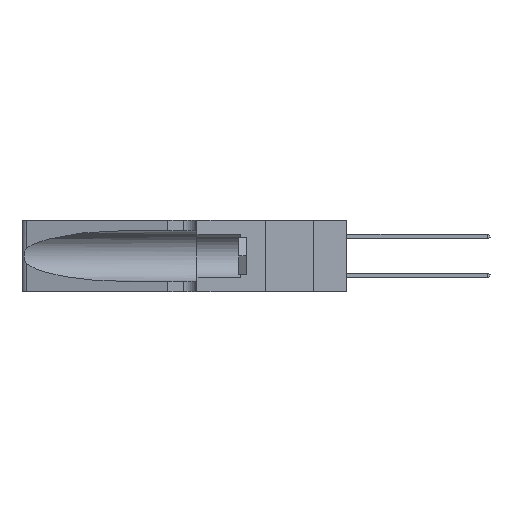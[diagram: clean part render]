
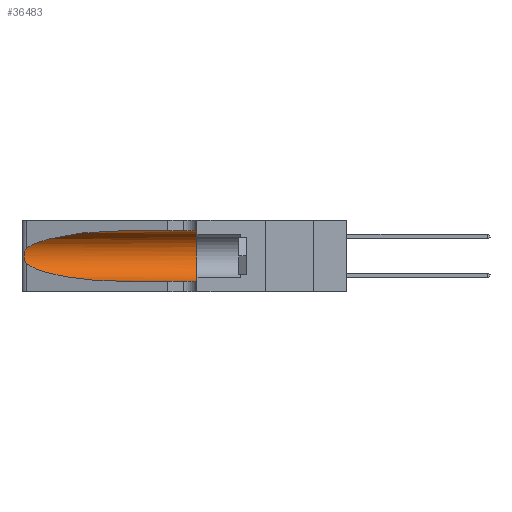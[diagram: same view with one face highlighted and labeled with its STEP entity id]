
A CAD part, left-side view. The second image highlights one B-rep face of the part: STEP entity #36483.
In plain terms, the highlighted cylindrical face has radius 3.308 mm (diameter 6.617 mm), a partial arc.
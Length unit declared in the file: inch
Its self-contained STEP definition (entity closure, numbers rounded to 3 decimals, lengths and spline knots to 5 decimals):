
#464 = CARTESIAN_POINT ( 'NONE',  ( 0.25787, 1.23484, 0.2124 ) ) ;
#1125 = EDGE_CURVE ( 'NONE', #40027, #24316, #21915, .T. ) ;
#1671 = DIRECTION ( 'NONE',  ( 0., 0., -1. ) ) ;
#1837 = CARTESIAN_POINT ( 'NONE',  ( 0.25487, 1.22718, 0.22369 ) ) ;
#2092 = ORIENTED_EDGE ( 'NONE', *, *, #38889, .T. ) ;
#2293 = CARTESIAN_POINT ( 'NONE',  ( 0.1305, 0.35, 0.31525 ) ) ;
#3446 = ORIENTED_EDGE ( 'NONE', *, *, #42935, .T. ) ;
#3939 = CARTESIAN_POINT ( 'NONE',  ( 0.26018, 1.23835, 0.19895 ) ) ;
#4341 = CARTESIAN_POINT ( 'NONE',  ( 0.18966, 0.96281, 0.05475 ) ) ;
#5694 = EDGE_CURVE ( 'NONE', #40027, #6744, #12491, .T. ) ;
#5858 = EDGE_LOOP ( 'NONE', ( #23459, #6784, #3446, #2092, #9388, #17272 ) ) ;
#5968 =( BOUNDED_CURVE ( )  B_SPLINE_CURVE ( 3, ( #17790, #37858, #4341, #27891 ),
 .UNSPECIFIED., .F., .T. ) 
 B_SPLINE_CURVE_WITH_KNOTS ( ( 4, 4 ),
 ( 3.44316, 4.71239 ),
 .UNSPECIFIED. ) 
 CURVE ( )  GEOMETRIC_REPRESENTATION_ITEM ( )  RATIONAL_B_SPLINE_CURVE ( ( 1., 0.87, 0.87, 1. ) ) 
 REPRESENTATION_ITEM ( '' )  );
#6744 = VERTEX_POINT ( 'NONE', #41160 ) ;
#6784 = ORIENTED_EDGE ( 'NONE', *, *, #17450, .T. ) ;
#7331 = VERTEX_POINT ( 'NONE', #17408 ) ;
#7383 = CARTESIAN_POINT ( 'NONE',  ( 0.26075, 1.23896, 0.178 ) ) ;
#9388 = ORIENTED_EDGE ( 'NONE', *, *, #13090, .F. ) ;
#10793 = CARTESIAN_POINT ( 'NONE',  ( 0.25856, 1.23593, 0.16098 ) ) ;
#11175 = CARTESIAN_POINT ( 'NONE',  ( 0.25487, 1.22718, 0.14631 ) ) ;
#12491 =( BOUNDED_CURVE ( )  B_SPLINE_CURVE ( 3, ( #22153, #35436, #28716, #1837 ),
 .UNSPECIFIED., .F., .F. ) 
 B_SPLINE_CURVE_WITH_KNOTS ( ( 4, 4 ),
 ( 1.5708, 2.84003 ),
 .UNSPECIFIED. ) 
 CURVE ( )  GEOMETRIC_REPRESENTATION_ITEM ( )  RATIONAL_B_SPLINE_CURVE ( ( 1., 0.87, 0.87, 1. ) ) 
 REPRESENTATION_ITEM ( '' )  );
#12757 = CARTESIAN_POINT ( 'NONE',  ( 0.1305, 0.35, 0.185 ) ) ;
#13090 = EDGE_CURVE ( 'NONE', #24316, #29160, #30477, .T. ) ;
#13878 = CARTESIAN_POINT ( 'NONE',  ( 0.1305, 1.61858, 0.31525 ) ) ;
#14041 = CYLINDRICAL_SURFACE ( 'NONE', #29720, 0.13025 ) ;
#14158 = CARTESIAN_POINT ( 'NONE',  ( 0.25639, 1.23186, 0.15144 ) ) ;
#14330 = VECTOR ( 'NONE', #26242, 39.37008 ) ;
#14621 = VERTEX_POINT ( 'NONE', #11175 ) ;
#15208 = DIRECTION ( 'NONE',  ( 0., -1., 0. ) ) ;
#15244 = CARTESIAN_POINT ( 'NONE',  ( 0.1305, 0.35, 0.05475 ) ) ;
#16123 = DIRECTION ( 'NONE',  ( 0., 0., 1. ) ) ;
#17130 = DIRECTION ( 'NONE',  ( 0., -1., 0. ) ) ;
#17272 = ORIENTED_EDGE ( 'NONE', *, *, #1125, .F. ) ;
#17408 = CARTESIAN_POINT ( 'NONE',  ( 0.1305, 0.72297, 0.05475 ) ) ;
#17410 = CARTESIAN_POINT ( 'NONE',  ( 0.25487, 1.22718, 0.22369 ) ) ;
#17450 = EDGE_CURVE ( 'NONE', #6744, #14621, #32653, .T. ) ;
#17561 = CARTESIAN_POINT ( 'NONE',  ( 0.25487, 1.22718, 0.14631 ) ) ;
#17790 = CARTESIAN_POINT ( 'NONE',  ( 0.25487, 1.22718, 0.14631 ) ) ;
#20792 = CARTESIAN_POINT ( 'NONE',  ( 0.25639, 1.23184, 0.21858 ) ) ;
#21655 = CARTESIAN_POINT ( 'NONE',  ( 0.1305, 0.72297, 0.31525 ) ) ;
#21915 = LINE ( 'NONE', #13878, #32929 ) ;
#21982 = CARTESIAN_POINT ( 'NONE',  ( 0.1305, 1.61858, 0.185 ) ) ;
#22153 = CARTESIAN_POINT ( 'NONE',  ( 0.1305, 0.72297, 0.31525 ) ) ;
#22919 = CARTESIAN_POINT ( 'NONE',  ( 0.1305, 1.61858, 0.05475 ) ) ;
#23459 = ORIENTED_EDGE ( 'NONE', *, *, #5694, .T. ) ;
#24155 = CARTESIAN_POINT ( 'NONE',  ( 0.25854, 1.2359, 0.20912 ) ) ;
#24316 = VERTEX_POINT ( 'NONE', #2293 ) ;
#26242 = DIRECTION ( 'NONE',  ( 0., -1., 0. ) ) ;
#27503 = CARTESIAN_POINT ( 'NONE',  ( 0.26075, 1.23896, 0.19203 ) ) ;
#27891 = CARTESIAN_POINT ( 'NONE',  ( 0.1305, 0.72297, 0.05475 ) ) ;
#28716 = CARTESIAN_POINT ( 'NONE',  ( 0.2373, 1.15595, 0.28018 ) ) ;
#29160 = VERTEX_POINT ( 'NONE', #15244 ) ;
#29720 = AXIS2_PLACEMENT_3D ( 'NONE', #21982, #15208, #1671 ) ;
#30477 = CIRCLE ( 'NONE', #31094, 0.13025 ) ;
#30759 = CARTESIAN_POINT ( 'NONE',  ( 0.25555, 1.22994, 0.2215 ) ) ;
#30891 = CARTESIAN_POINT ( 'NONE',  ( 0.26017, 1.23833, 0.17102 ) ) ;
#31094 = AXIS2_PLACEMENT_3D ( 'NONE', #12757, #36186, #16123 ) ;
#31896 = FACE_OUTER_BOUND ( 'NONE', #5858, .T. ) ;
#32653 = B_SPLINE_CURVE_WITH_KNOTS ( 'NONE', 3,
 ( #17410, #30759, #20792, #464, #24155, #3939, #27503, #7383, #30891, #10793, #34248, #14158, #37618, #17561 ),
 .UNSPECIFIED., .F., .F.,
 ( 4, 2, 2, 2, 2, 2, 4 ),
 ( 0., 0.00027, 0.00053, 0.00107, 0.0016, 0.00187, 0.00214 ),
 .UNSPECIFIED. ) ;
#32929 = VECTOR ( 'NONE', #17130, 39.37008 ) ;
#34248 = CARTESIAN_POINT ( 'NONE',  ( 0.25789, 1.23486, 0.15765 ) ) ;
#35436 = CARTESIAN_POINT ( 'NONE',  ( 0.18966, 0.96281, 0.31525 ) ) ;
#36186 = DIRECTION ( 'NONE',  ( 0., 1., 0. ) ) ;
#36483 = ADVANCED_FACE ( 'NONE', ( #31896 ), #14041, .F. ) ;
#37618 = CARTESIAN_POINT ( 'NONE',  ( 0.25555, 1.22993, 0.14849 ) ) ;
#37858 = CARTESIAN_POINT ( 'NONE',  ( 0.2373, 1.15595, 0.08982 ) ) ;
#38889 = EDGE_CURVE ( 'NONE', #7331, #29160, #41080, .T. ) ;
#40027 = VERTEX_POINT ( 'NONE', #21655 ) ;
#41080 = LINE ( 'NONE', #22919, #14330 ) ;
#41160 = CARTESIAN_POINT ( 'NONE',  ( 0.25487, 1.22718, 0.22369 ) ) ;
#42935 = EDGE_CURVE ( 'NONE', #14621, #7331, #5968, .T. ) ;
